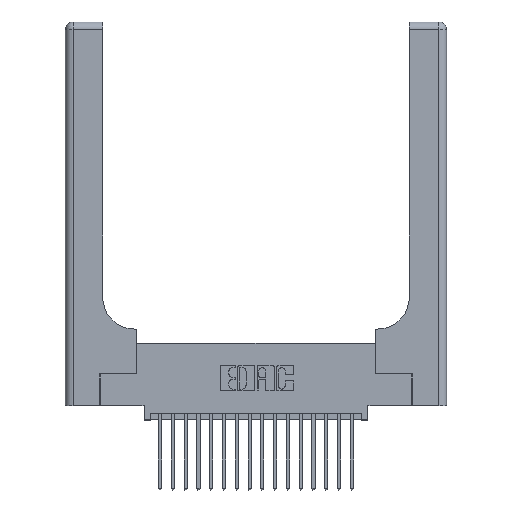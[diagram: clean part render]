
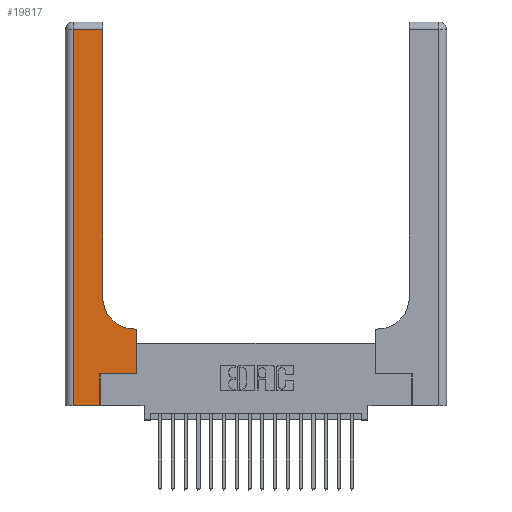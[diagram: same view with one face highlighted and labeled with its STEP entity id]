
A CAD part, top view. The second image highlights one B-rep face of the part: STEP entity #19817.
In plain terms, the highlighted planar face has unit normal (0, 0, 1).
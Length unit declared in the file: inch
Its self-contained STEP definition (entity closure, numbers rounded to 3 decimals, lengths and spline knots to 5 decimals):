
#11 = VERTEX_POINT ( 'NONE', #11457 ) ;
#195 = EDGE_CURVE ( 'NONE', #1441, #4255, #14832, .T. ) ;
#483 = DIRECTION ( 'NONE',  ( -1., 0., 0. ) ) ;
#490 = LINE ( 'NONE', #9134, #17712 ) ;
#1023 = AXIS2_PLACEMENT_3D ( 'NONE', #13824, #3865, #15447 ) ;
#1216 = DIRECTION ( 'NONE',  ( 0., 1., 0. ) ) ;
#1341 = VECTOR ( 'NONE', #2344, 39.37008 ) ;
#1398 = VERTEX_POINT ( 'NONE', #10798 ) ;
#1441 = VERTEX_POINT ( 'NONE', #7944 ) ;
#1712 = ORIENTED_EDGE ( 'NONE', *, *, #16882, .T. ) ;
#2231 = LINE ( 'NONE', #16260, #6825 ) ;
#2344 = DIRECTION ( 'NONE',  ( -1., 0., 0. ) ) ;
#2481 = VECTOR ( 'NONE', #8429, 39.37008 ) ;
#2960 = CARTESIAN_POINT ( 'NONE',  ( 0.2915, 0.6, 0.37 ) ) ;
#3865 = DIRECTION ( 'NONE',  ( 0., 0., -1. ) ) ;
#4064 = DIRECTION ( 'NONE',  ( 1., 0., 0. ) ) ;
#4255 = VERTEX_POINT ( 'NONE', #5894 ) ;
#4363 = VECTOR ( 'NONE', #20670, 39.37008 ) ;
#5036 = EDGE_CURVE ( 'NONE', #14428, #20520, #16356, .T. ) ;
#5894 = CARTESIAN_POINT ( 'NONE',  ( 0.06, 0., 0.37 ) ) ;
#5985 = CARTESIAN_POINT ( 'NONE',  ( 0.5585, 0.25, 0.37 ) ) ;
#6638 = EDGE_CURVE ( 'NONE', #6858, #12871, #8958, .T. ) ;
#6825 = VECTOR ( 'NONE', #1216, 39.37008 ) ;
#6858 = VERTEX_POINT ( 'NONE', #14305 ) ;
#7439 = CARTESIAN_POINT ( 'NONE',  ( 0.5585, 0.6, 0.37 ) ) ;
#7701 = VECTOR ( 'NONE', #19583, 39.37008 ) ;
#7717 = AXIS2_PLACEMENT_3D ( 'NONE', #9022, #10773, #483 ) ;
#7733 = CARTESIAN_POINT ( 'NONE',  ( 0.06, 3., 0.37 ) ) ;
#7759 = DIRECTION ( 'NONE',  ( 0., -1., 0. ) ) ;
#7944 = CARTESIAN_POINT ( 'NONE',  ( 0.06, 2.94, 0.37 ) ) ;
#8429 = DIRECTION ( 'NONE',  ( 0., 1., 0. ) ) ;
#8601 = ORIENTED_EDGE ( 'NONE', *, *, #19246, .T. ) ;
#8958 = CIRCLE ( 'NONE', #1023, 0.25 ) ;
#9022 = CARTESIAN_POINT ( 'NONE',  ( 0., 3., 0.37 ) ) ;
#9102 = PLANE ( 'NONE',  #7717 ) ;
#9134 = CARTESIAN_POINT ( 'NONE',  ( 0., 0., 0.37 ) ) ;
#9482 = CARTESIAN_POINT ( 'NONE',  ( 0.269, 0.25, 0.37 ) ) ;
#10404 = ORIENTED_EDGE ( 'NONE', *, *, #12667, .T. ) ;
#10556 = ORIENTED_EDGE ( 'NONE', *, *, #12581, .T. ) ;
#10629 = ORIENTED_EDGE ( 'NONE', *, *, #6638, .T. ) ;
#10773 = DIRECTION ( 'NONE',  ( 0., 0., -1. ) ) ;
#10798 = CARTESIAN_POINT ( 'NONE',  ( 0.2915, 2.94, 0.37 ) ) ;
#10984 = EDGE_CURVE ( 'NONE', #18304, #11, #2231, .T. ) ;
#11457 = CARTESIAN_POINT ( 'NONE',  ( 0.269, 0.25, 0.37 ) ) ;
#11607 = VECTOR ( 'NONE', #7759, 39.37008 ) ;
#11657 = CARTESIAN_POINT ( 'NONE',  ( 0.5585, 0.25, 0.37 ) ) ;
#11659 = EDGE_CURVE ( 'NONE', #12871, #1398, #18982, .T. ) ;
#11689 = CARTESIAN_POINT ( 'NONE',  ( 0.2915, 0.85, 0.37 ) ) ;
#11953 = FACE_OUTER_BOUND ( 'NONE', #19594, .T. ) ;
#12125 = ORIENTED_EDGE ( 'NONE', *, *, #11659, .T. ) ;
#12332 = LINE ( 'NONE', #2960, #16574 ) ;
#12581 = EDGE_CURVE ( 'NONE', #1398, #1441, #14716, .T. ) ;
#12667 = EDGE_CURVE ( 'NONE', #11, #14428, #16973, .T. ) ;
#12871 = VERTEX_POINT ( 'NONE', #11689 ) ;
#12965 = ORIENTED_EDGE ( 'NONE', *, *, #10984, .T. ) ;
#13824 = CARTESIAN_POINT ( 'NONE',  ( 0.5415, 0.85, 0.37 ) ) ;
#14052 = ORIENTED_EDGE ( 'NONE', *, *, #5036, .T. ) ;
#14305 = CARTESIAN_POINT ( 'NONE',  ( 0.5415, 0.6, 0.37 ) ) ;
#14428 = VERTEX_POINT ( 'NONE', #5985 ) ;
#14609 = DIRECTION ( 'NONE',  ( -1., 0., 0. ) ) ;
#14684 = CARTESIAN_POINT ( 'NONE',  ( 0.269, 0., 0.37 ) ) ;
#14716 = LINE ( 'NONE', #15672, #1341 ) ;
#14832 = LINE ( 'NONE', #7733, #11607 ) ;
#15447 = DIRECTION ( 'NONE',  ( 1., 0., 0. ) ) ;
#15672 = CARTESIAN_POINT ( 'NONE',  ( 0., 2.94, 0.37 ) ) ;
#16089 = ORIENTED_EDGE ( 'NONE', *, *, #195, .T. ) ;
#16260 = CARTESIAN_POINT ( 'NONE',  ( 0.269, 0., 0.37 ) ) ;
#16356 = LINE ( 'NONE', #11657, #7701 ) ;
#16574 = VECTOR ( 'NONE', #14609, 39.37008 ) ;
#16882 = EDGE_CURVE ( 'NONE', #20520, #6858, #12332, .T. ) ;
#16973 = LINE ( 'NONE', #9482, #4363 ) ;
#17712 = VECTOR ( 'NONE', #4064, 39.37008 ) ;
#18088 = CARTESIAN_POINT ( 'NONE',  ( 0.2915, 3., 0.37 ) ) ;
#18304 = VERTEX_POINT ( 'NONE', #14684 ) ;
#18982 = LINE ( 'NONE', #18088, #2481 ) ;
#19246 = EDGE_CURVE ( 'NONE', #4255, #18304, #490, .T. ) ;
#19583 = DIRECTION ( 'NONE',  ( 0., 1., 0. ) ) ;
#19594 = EDGE_LOOP ( 'NONE', ( #12125, #10556, #16089, #8601, #12965, #10404, #14052, #1712, #10629 ) ) ;
#19817 = ADVANCED_FACE ( 'NONE', ( #11953 ), #9102, .F. ) ;
#20520 = VERTEX_POINT ( 'NONE', #7439 ) ;
#20670 = DIRECTION ( 'NONE',  ( 1., 0., 0. ) ) ;
